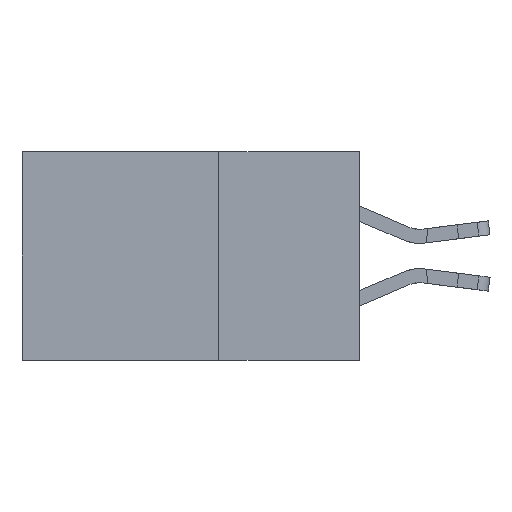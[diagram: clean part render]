
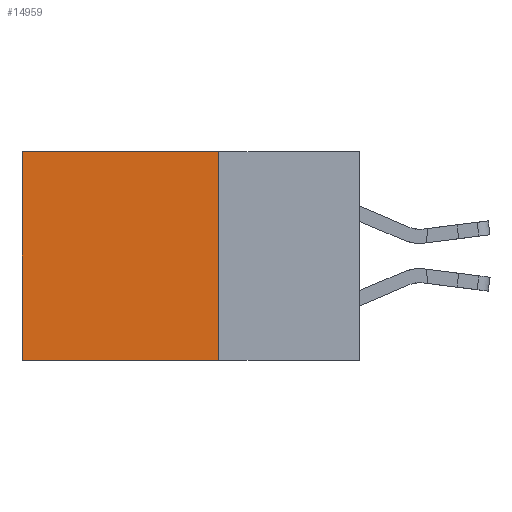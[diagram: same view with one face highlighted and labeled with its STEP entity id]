
A CAD part, left-side view. The second image highlights one B-rep face of the part: STEP entity #14959.
In plain terms, the highlighted planar face has unit normal (-1, 0, 0).
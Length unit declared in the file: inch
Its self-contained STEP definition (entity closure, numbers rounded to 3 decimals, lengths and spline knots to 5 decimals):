
#346 = CARTESIAN_POINT ( 'NONE',  ( 0.2875, 0.25, 0. ) ) ;
#1057 = LINE ( 'NONE', #8366, #1497 ) ;
#1497 = VECTOR ( 'NONE', #14369, 39.37008 ) ;
#1732 = DIRECTION ( 'NONE',  ( 0., 1., 0. ) ) ;
#2144 = ORIENTED_EDGE ( 'NONE', *, *, #2593, .F. ) ;
#2593 = EDGE_CURVE ( 'NONE', #16281, #18607, #17795, .T. ) ;
#2994 = VERTEX_POINT ( 'NONE', #16384 ) ;
#3233 = VECTOR ( 'NONE', #1732, 39.37008 ) ;
#3637 = AXIS2_PLACEMENT_3D ( 'NONE', #346, #4663, #11999 ) ;
#4276 = EDGE_CURVE ( 'NONE', #16281, #2994, #1057, .T. ) ;
#4663 = DIRECTION ( 'NONE',  ( 1., 0., 0. ) ) ;
#6867 = EDGE_CURVE ( 'NONE', #2994, #18275, #17158, .T. ) ;
#8060 = DIRECTION ( 'NONE',  ( 0., 0., -1. ) ) ;
#8062 = CARTESIAN_POINT ( 'NONE',  ( 0.2875, 0.25, 0. ) ) ;
#8366 = CARTESIAN_POINT ( 'NONE',  ( 0.2875, 0.25, 0. ) ) ;
#9152 = CARTESIAN_POINT ( 'NONE',  ( 0.2875, 0.6, 0. ) ) ;
#11999 = DIRECTION ( 'NONE',  ( 0., 0., -1. ) ) ;
#12076 = LINE ( 'NONE', #15072, #3233 ) ;
#12389 = EDGE_CURVE ( 'NONE', #18607, #18275, #12076, .T. ) ;
#12708 = CARTESIAN_POINT ( 'NONE',  ( 0.2875, 0.25, -0.37 ) ) ;
#13182 = VECTOR ( 'NONE', #8060, 39.37008 ) ;
#13484 = DIRECTION ( 'NONE',  ( 0., 0., -1. ) ) ;
#13848 = CARTESIAN_POINT ( 'NONE',  ( 0.2875, 0.25, 0. ) ) ;
#14117 = ORIENTED_EDGE ( 'NONE', *, *, #4276, .T. ) ;
#14369 = DIRECTION ( 'NONE',  ( 0., 1., 0. ) ) ;
#14382 = ORIENTED_EDGE ( 'NONE', *, *, #6867, .T. ) ;
#14655 = EDGE_LOOP ( 'NONE', ( #14382, #18367, #2144, #14117 ) ) ;
#14959 = ADVANCED_FACE ( 'NONE', ( #15168 ), #16238, .F. ) ;
#14965 = CARTESIAN_POINT ( 'NONE',  ( 0.2875, 0.6, -0.37 ) ) ;
#15072 = CARTESIAN_POINT ( 'NONE',  ( 0.2875, 0.25, -0.37 ) ) ;
#15168 = FACE_OUTER_BOUND ( 'NONE', #14655, .T. ) ;
#16238 = PLANE ( 'NONE',  #3637 ) ;
#16281 = VERTEX_POINT ( 'NONE', #8062 ) ;
#16384 = CARTESIAN_POINT ( 'NONE',  ( 0.2875, 0.6, 0. ) ) ;
#17158 = LINE ( 'NONE', #9152, #17393 ) ;
#17393 = VECTOR ( 'NONE', #13484, 39.37008 ) ;
#17795 = LINE ( 'NONE', #13848, #13182 ) ;
#18275 = VERTEX_POINT ( 'NONE', #14965 ) ;
#18367 = ORIENTED_EDGE ( 'NONE', *, *, #12389, .F. ) ;
#18607 = VERTEX_POINT ( 'NONE', #12708 ) ;
